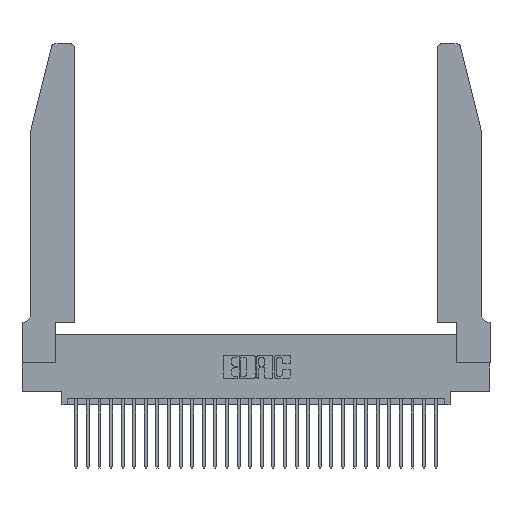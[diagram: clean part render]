
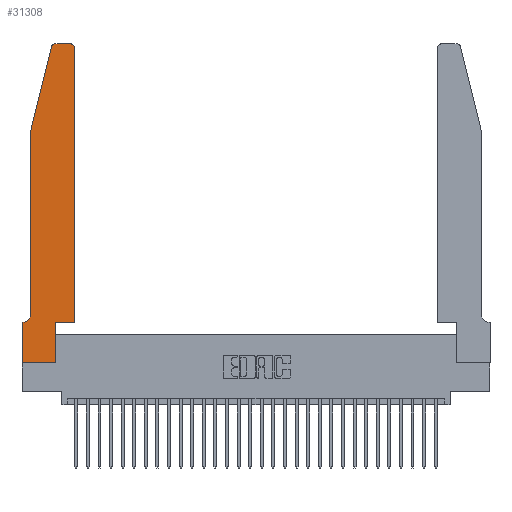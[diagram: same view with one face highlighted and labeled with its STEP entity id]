
A CAD part, top view. The second image highlights one B-rep face of the part: STEP entity #31308.
In plain terms, the highlighted planar face has unit normal (0, 0, 1).
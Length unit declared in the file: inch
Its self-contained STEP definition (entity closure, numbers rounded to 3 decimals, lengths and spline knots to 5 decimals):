
#55 = CARTESIAN_POINT ( 'NONE',  ( 0.284, 2.72, 0.37 ) ) ;
#129 = DIRECTION ( 'NONE',  ( -1., 0., 0. ) ) ;
#156 = DIRECTION ( 'NONE',  ( 1., 0., 0. ) ) ;
#266 = CARTESIAN_POINT ( 'NONE',  ( 0., 0.35, 0.37 ) ) ;
#283 = DIRECTION ( 'NONE',  ( 0., 1., 0. ) ) ;
#1492 = VERTEX_POINT ( 'NONE', #5896 ) ;
#1762 = CARTESIAN_POINT ( 'NONE',  ( 0.0755, 0.42, 0.37 ) ) ;
#1763 = EDGE_CURVE ( 'NONE', #22468, #21894, #30249, .T. ) ;
#1991 = DIRECTION ( 'NONE',  ( 1., 0., 0. ) ) ;
#2239 = CARTESIAN_POINT ( 'NONE',  ( 0., 0., 0.37 ) ) ;
#2292 = ORIENTED_EDGE ( 'NONE', *, *, #1763, .T. ) ;
#2349 = CARTESIAN_POINT ( 'NONE',  ( 0., 0., 0.37 ) ) ;
#2457 = EDGE_CURVE ( 'NONE', #28721, #15339, #29142, .T. ) ;
#2461 = EDGE_CURVE ( 'NONE', #19668, #28721, #21153, .T. ) ;
#2610 = CARTESIAN_POINT ( 'NONE',  ( 0.2865, 0.35, 0.37 ) ) ;
#2935 = DIRECTION ( 'NONE',  ( -1., 0., 0. ) ) ;
#3055 = VERTEX_POINT ( 'NONE', #15172 ) ;
#3079 = AXIS2_PLACEMENT_3D ( 'NONE', #11450, #21000, #18768 ) ;
#3149 = CARTESIAN_POINT ( 'NONE',  ( 0.0055, 0.42, 0.37 ) ) ;
#3303 = DIRECTION ( 'NONE',  ( 0., -1., 0. ) ) ;
#3395 = LINE ( 'NONE', #2349, #16640 ) ;
#3877 = CARTESIAN_POINT ( 'NONE',  ( 0.4505, 0.35, 0.37 ) ) ;
#5077 = ORIENTED_EDGE ( 'NONE', *, *, #10432, .T. ) ;
#5611 = LINE ( 'NONE', #6848, #26878 ) ;
#5618 = CARTESIAN_POINT ( 'NONE',  ( 0.0755, 2., 0.37 ) ) ;
#5635 = ORIENTED_EDGE ( 'NONE', *, *, #14078, .T. ) ;
#5896 = CARTESIAN_POINT ( 'NONE',  ( 0.4505, 2.72, 0.37 ) ) ;
#6848 = CARTESIAN_POINT ( 'NONE',  ( 0.4505, 0.35, 0.37 ) ) ;
#7276 = CARTESIAN_POINT ( 'NONE',  ( 0.2865, 0., 0.37 ) ) ;
#7529 = CARTESIAN_POINT ( 'NONE',  ( 0.2605, 2.75, 0.37 ) ) ;
#7777 = DIRECTION ( 'NONE',  ( -0.239, -0.971, 0. ) ) ;
#7898 = DIRECTION ( 'NONE',  ( 0., 0., -1. ) ) ;
#8528 = LINE ( 'NONE', #7529, #30512 ) ;
#8825 = VERTEX_POINT ( 'NONE', #2239 ) ;
#9429 = DIRECTION ( 'NONE',  ( 0., -1., 0. ) ) ;
#9703 = CARTESIAN_POINT ( 'NONE',  ( 0., 0., 0.37 ) ) ;
#10051 = DIRECTION ( 'NONE',  ( -1., 0., 0. ) ) ;
#10432 = EDGE_CURVE ( 'NONE', #3055, #1492, #5611, .T. ) ;
#10947 = ORIENTED_EDGE ( 'NONE', *, *, #29423, .T. ) ;
#11384 = VERTEX_POINT ( 'NONE', #26978 ) ;
#11395 = ORIENTED_EDGE ( 'NONE', *, *, #30018, .T. ) ;
#11450 = CARTESIAN_POINT ( 'NONE',  ( 0.4205, 2.72, 0.37 ) ) ;
#11764 = CIRCLE ( 'NONE', #18299, 0.03 ) ;
#11846 = EDGE_LOOP ( 'NONE', ( #11395, #17329, #10947, #14316, #12339, #25871, #22062, #18980, #2292, #5635, #5077, #23668 ) ) ;
#11980 = CARTESIAN_POINT ( 'NONE',  ( 0.284, 2.75, 0.37 ) ) ;
#12339 = ORIENTED_EDGE ( 'NONE', *, *, #2461, .T. ) ;
#12854 = CARTESIAN_POINT ( 'NONE',  ( 0.0755, 2., 0.37 ) ) ;
#13505 = VECTOR ( 'NONE', #7777, 39.37008 ) ;
#14078 = EDGE_CURVE ( 'NONE', #21894, #3055, #17888, .T. ) ;
#14316 = ORIENTED_EDGE ( 'NONE', *, *, #17701, .T. ) ;
#14327 = EDGE_CURVE ( 'NONE', #8825, #22468, #24714, .T. ) ;
#14393 = LINE ( 'NONE', #5618, #23890 ) ;
#15099 = AXIS2_PLACEMENT_3D ( 'NONE', #3149, #7898, #2935 ) ;
#15172 = CARTESIAN_POINT ( 'NONE',  ( 0.4505, 0.35, 0.37 ) ) ;
#15339 = VERTEX_POINT ( 'NONE', #30759 ) ;
#16640 = VECTOR ( 'NONE', #9429, 39.37008 ) ;
#17329 = ORIENTED_EDGE ( 'NONE', *, *, #26652, .T. ) ;
#17360 = VECTOR ( 'NONE', #283, 39.37008 ) ;
#17701 = EDGE_CURVE ( 'NONE', #11384, #19668, #14393, .T. ) ;
#17888 = LINE ( 'NONE', #3877, #23572 ) ;
#18016 = EDGE_CURVE ( 'NONE', #15339, #8825, #3395, .T. ) ;
#18191 = CIRCLE ( 'NONE', #3079, 0.03 ) ;
#18299 = AXIS2_PLACEMENT_3D ( 'NONE', #55, #24114, #1991 ) ;
#18768 = DIRECTION ( 'NONE',  ( 1., 0., 0. ) ) ;
#18841 = DIRECTION ( 'NONE',  ( 0., 1., 0. ) ) ;
#18980 = ORIENTED_EDGE ( 'NONE', *, *, #14327, .T. ) ;
#18988 = AXIS2_PLACEMENT_3D ( 'NONE', #266, #19856, #156 ) ;
#19360 = CARTESIAN_POINT ( 'NONE',  ( 0.0055, 0.35, 0.37 ) ) ;
#19532 = DIRECTION ( 'NONE',  ( 1., 0., 0. ) ) ;
#19668 = VERTEX_POINT ( 'NONE', #1762 ) ;
#19856 = DIRECTION ( 'NONE',  ( 0., 0., 1. ) ) ;
#20830 = DIRECTION ( 'NONE',  ( 1., 0., 0. ) ) ;
#21000 = DIRECTION ( 'NONE',  ( 0., 0., 1. ) ) ;
#21153 = CIRCLE ( 'NONE', #15099, 0.07 ) ;
#21894 = VERTEX_POINT ( 'NONE', #24169 ) ;
#22062 = ORIENTED_EDGE ( 'NONE', *, *, #18016, .T. ) ;
#22468 = VERTEX_POINT ( 'NONE', #7276 ) ;
#22606 = LINE ( 'NONE', #12854, #13505 ) ;
#22758 = VERTEX_POINT ( 'NONE', #29950 ) ;
#23572 = VECTOR ( 'NONE', #20830, 39.37008 ) ;
#23668 = ORIENTED_EDGE ( 'NONE', *, *, #27039, .T. ) ;
#23890 = VECTOR ( 'NONE', #3303, 39.37008 ) ;
#24114 = DIRECTION ( 'NONE',  ( 0., 0., 1. ) ) ;
#24169 = CARTESIAN_POINT ( 'NONE',  ( 0.2865, 0.35, 0.37 ) ) ;
#24475 = CARTESIAN_POINT ( 'NONE',  ( 0.25487, 2.72718, 0.37 ) ) ;
#24714 = LINE ( 'NONE', #9703, #26234 ) ;
#25344 = VERTEX_POINT ( 'NONE', #11980 ) ;
#25871 = ORIENTED_EDGE ( 'NONE', *, *, #2457, .T. ) ;
#26047 = VERTEX_POINT ( 'NONE', #24475 ) ;
#26101 = VECTOR ( 'NONE', #10051, 39.37008 ) ;
#26234 = VECTOR ( 'NONE', #19532, 39.37008 ) ;
#26652 = EDGE_CURVE ( 'NONE', #25344, #26047, #11764, .T. ) ;
#26878 = VECTOR ( 'NONE', #18841, 39.37008 ) ;
#26978 = CARTESIAN_POINT ( 'NONE',  ( 0.0755, 2., 0.37 ) ) ;
#27039 = EDGE_CURVE ( 'NONE', #1492, #22758, #18191, .T. ) ;
#28721 = VERTEX_POINT ( 'NONE', #19360 ) ;
#29142 = LINE ( 'NONE', #29653, #26101 ) ;
#29314 = FACE_OUTER_BOUND ( 'NONE', #11846, .T. ) ;
#29423 = EDGE_CURVE ( 'NONE', #26047, #11384, #22606, .T. ) ;
#29509 = PLANE ( 'NONE',  #18988 ) ;
#29653 = CARTESIAN_POINT ( 'NONE',  ( 0.0755, 0.35, 0.37 ) ) ;
#29950 = CARTESIAN_POINT ( 'NONE',  ( 0.4205, 2.75, 0.37 ) ) ;
#30018 = EDGE_CURVE ( 'NONE', #22758, #25344, #8528, .T. ) ;
#30249 = LINE ( 'NONE', #2610, #17360 ) ;
#30512 = VECTOR ( 'NONE', #129, 39.37008 ) ;
#30759 = CARTESIAN_POINT ( 'NONE',  ( 0., 0.35, 0.37 ) ) ;
#31308 = ADVANCED_FACE ( 'NONE', ( #29314 ), #29509, .T. ) ;
